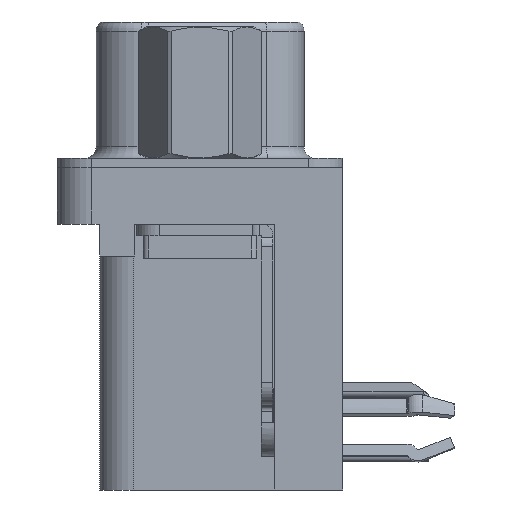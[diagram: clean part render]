
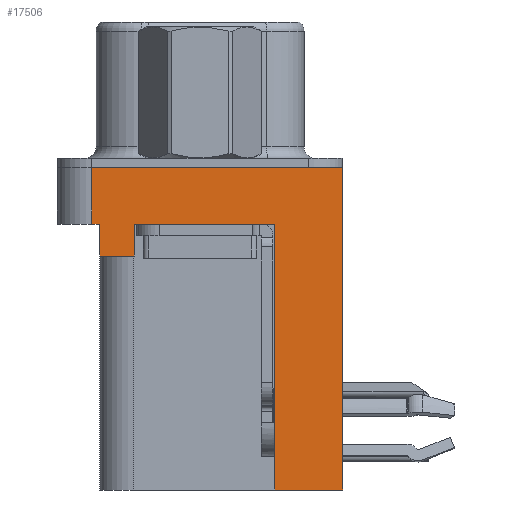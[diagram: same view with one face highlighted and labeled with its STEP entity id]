
A CAD part, left-side view. The second image highlights one B-rep face of the part: STEP entity #17506.
In plain terms, the highlighted planar face has unit normal (-1, 0, 0).
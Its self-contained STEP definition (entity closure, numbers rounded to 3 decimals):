
#22 = DIRECTION ( 'NONE',  ( 0., -1., 0. ) ) ;
#351 = DIRECTION ( 'NONE',  ( 0., 0., 1. ) ) ;
#468 = DIRECTION ( 'NONE',  ( 0., -1., 0. ) ) ;
#763 = DIRECTION ( 'NONE',  ( 0., 0., 1. ) ) ;
#783 = ORIENTED_EDGE ( 'NONE', *, *, #10954, .F. ) ;
#918 = LINE ( 'NONE', #12548, #12330 ) ;
#1053 = VECTOR ( 'NONE', #14538, 1000. ) ;
#1169 = ORIENTED_EDGE ( 'NONE', *, *, #12065, .F. ) ;
#1178 = DIRECTION ( 'NONE',  ( 0., 0., 1. ) ) ;
#1219 = ORIENTED_EDGE ( 'NONE', *, *, #16926, .F. ) ;
#1365 = VERTEX_POINT ( 'NONE', #20836 ) ;
#1404 = EDGE_LOOP ( 'NONE', ( #9701, #24889, #11988, #1169, #1219, #25271, #9842, #10810, #783, #14879 ) ) ;
#1715 = CARTESIAN_POINT ( 'NONE',  ( -2.935, 4.425, -3.9 ) ) ;
#1854 = VERTEX_POINT ( 'NONE', #5309 ) ;
#2257 = VERTEX_POINT ( 'NONE', #22942 ) ;
#2873 = AXIS2_PLACEMENT_3D ( 'NONE', #8880, #4756, #763 ) ;
#3659 = VECTOR ( 'NONE', #25088, 1000. ) ;
#3958 = CARTESIAN_POINT ( 'NONE',  ( -2.935, -6.275, -2.5 ) ) ;
#4233 = VECTOR ( 'NONE', #22351, 1000. ) ;
#4756 = DIRECTION ( 'NONE',  ( -1., 0., 0. ) ) ;
#4772 = DIRECTION ( 'NONE',  ( 0., 0., 1. ) ) ;
#5073 = VERTEX_POINT ( 'NONE', #14585 ) ;
#5309 = CARTESIAN_POINT ( 'NONE',  ( -2.935, -3.295, -2.5 ) ) ;
#5387 = CARTESIAN_POINT ( 'NONE',  ( -2.935, 4.425, -3.9 ) ) ;
#5427 = VERTEX_POINT ( 'NONE', #12241 ) ;
#5626 = VECTOR ( 'NONE', #351, 1000. ) ;
#5876 = EDGE_CURVE ( 'NONE', #1365, #6861, #22966, .T. ) ;
#6420 = CARTESIAN_POINT ( 'NONE',  ( -2.935, -3.295, -14.2 ) ) ;
#6432 = VERTEX_POINT ( 'NONE', #11046 ) ;
#6572 = FACE_OUTER_BOUND ( 'NONE', #1404, .T. ) ;
#6861 = VERTEX_POINT ( 'NONE', #15035 ) ;
#6999 = LINE ( 'NONE', #11243, #17863 ) ;
#7480 = LINE ( 'NONE', #3958, #18390 ) ;
#8097 = EDGE_CURVE ( 'NONE', #21953, #2257, #6999, .T. ) ;
#8880 = CARTESIAN_POINT ( 'NONE',  ( -2.935, -6.275, -2.5 ) ) ;
#9420 = DIRECTION ( 'NONE',  ( 0., 0., 1. ) ) ;
#9701 = ORIENTED_EDGE ( 'NONE', *, *, #10959, .F. ) ;
#9842 = ORIENTED_EDGE ( 'NONE', *, *, #22201, .T. ) ;
#10077 = CARTESIAN_POINT ( 'NONE',  ( -2.935, -6.275, 0. ) ) ;
#10462 = LINE ( 'NONE', #12788, #4233 ) ;
#10793 = EDGE_CURVE ( 'NONE', #5073, #14173, #7480, .T. ) ;
#10810 = ORIENTED_EDGE ( 'NONE', *, *, #17257, .F. ) ;
#10954 = EDGE_CURVE ( 'NONE', #5073, #5427, #20351, .T. ) ;
#10959 = EDGE_CURVE ( 'NONE', #2257, #14173, #22408, .T. ) ;
#11046 = CARTESIAN_POINT ( 'NONE',  ( -2.935, 4.425, -3.9 ) ) ;
#11243 = CARTESIAN_POINT ( 'NONE',  ( -2.935, 4.775, -2.5 ) ) ;
#11314 = CARTESIAN_POINT ( 'NONE',  ( -2.935, 4.775, -2.5 ) ) ;
#11988 = ORIENTED_EDGE ( 'NONE', *, *, #25534, .T. ) ;
#12065 = EDGE_CURVE ( 'NONE', #6432, #22928, #17159, .T. ) ;
#12241 = CARTESIAN_POINT ( 'NONE',  ( -2.935, -3.295, -14.2 ) ) ;
#12330 = VECTOR ( 'NONE', #1178, 1000. ) ;
#12548 = CARTESIAN_POINT ( 'NONE',  ( -2.935, -3.295, -14.2 ) ) ;
#12788 = CARTESIAN_POINT ( 'NONE',  ( -2.935, -6.275, -2.5 ) ) ;
#14173 = VERTEX_POINT ( 'NONE', #10077 ) ;
#14538 = DIRECTION ( 'NONE',  ( 0., 1., 0. ) ) ;
#14585 = CARTESIAN_POINT ( 'NONE',  ( -2.935, -6.275, -14.2 ) ) ;
#14841 = CARTESIAN_POINT ( 'NONE',  ( -2.935, 2.895, -3.9 ) ) ;
#14879 = ORIENTED_EDGE ( 'NONE', *, *, #10793, .T. ) ;
#15035 = CARTESIAN_POINT ( 'NONE',  ( -2.935, 2.895, -2.5 ) ) ;
#15656 = LINE ( 'NONE', #23511, #23746 ) ;
#16926 = EDGE_CURVE ( 'NONE', #1365, #6432, #17224, .T. ) ;
#17159 = LINE ( 'NONE', #5387, #5626 ) ;
#17224 = LINE ( 'NONE', #1715, #3659 ) ;
#17257 = EDGE_CURVE ( 'NONE', #5427, #1854, #918, .T. ) ;
#17506 = ADVANCED_FACE ( 'NONE', ( #6572 ), #22320, .T. ) ;
#17863 = VECTOR ( 'NONE', #18997, 1000. ) ;
#18390 = VECTOR ( 'NONE', #9420, 1000. ) ;
#18997 = DIRECTION ( 'NONE',  ( 0., 0., 1. ) ) ;
#20351 = LINE ( 'NONE', #6420, #1053 ) ;
#20446 = VECTOR ( 'NONE', #468, 1000. ) ;
#20836 = CARTESIAN_POINT ( 'NONE',  ( -2.935, 2.895, -3.9 ) ) ;
#21953 = VERTEX_POINT ( 'NONE', #11314 ) ;
#22201 = EDGE_CURVE ( 'NONE', #6861, #1854, #10462, .T. ) ;
#22285 = CARTESIAN_POINT ( 'NONE',  ( -2.935, -6.275, 0. ) ) ;
#22320 = PLANE ( 'NONE',  #2873 ) ;
#22351 = DIRECTION ( 'NONE',  ( 0., -1., 0. ) ) ;
#22408 = LINE ( 'NONE', #22285, #20446 ) ;
#22928 = VERTEX_POINT ( 'NONE', #23819 ) ;
#22942 = CARTESIAN_POINT ( 'NONE',  ( -2.935, 4.775, 0. ) ) ;
#22966 = LINE ( 'NONE', #14841, #24036 ) ;
#23511 = CARTESIAN_POINT ( 'NONE',  ( -2.935, -6.275, -2.5 ) ) ;
#23746 = VECTOR ( 'NONE', #22, 1000. ) ;
#23819 = CARTESIAN_POINT ( 'NONE',  ( -2.935, 4.425, -2.5 ) ) ;
#24036 = VECTOR ( 'NONE', #4772, 1000. ) ;
#24889 = ORIENTED_EDGE ( 'NONE', *, *, #8097, .F. ) ;
#25088 = DIRECTION ( 'NONE',  ( 0., 1., 0. ) ) ;
#25271 = ORIENTED_EDGE ( 'NONE', *, *, #5876, .T. ) ;
#25534 = EDGE_CURVE ( 'NONE', #21953, #22928, #15656, .T. ) ;
